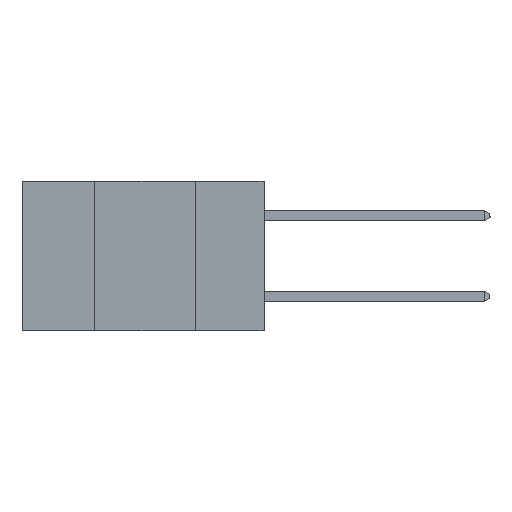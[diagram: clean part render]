
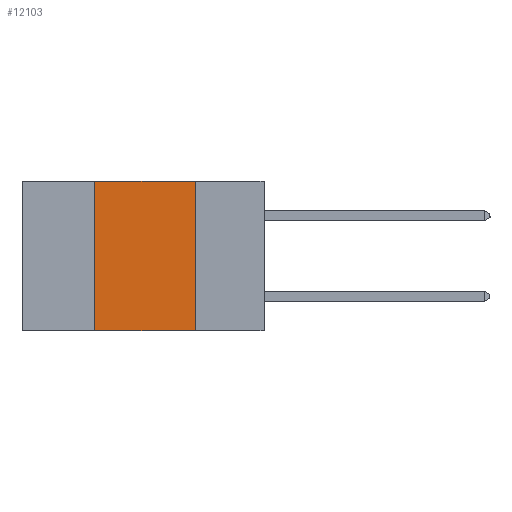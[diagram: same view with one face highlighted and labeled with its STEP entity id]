
A CAD part, left-side view. The second image highlights one B-rep face of the part: STEP entity #12103.
In plain terms, the highlighted planar face has unit normal (-1, 0, 0).
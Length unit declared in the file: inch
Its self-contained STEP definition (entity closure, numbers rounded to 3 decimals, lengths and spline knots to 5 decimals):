
#478 = EDGE_CURVE ( 'NONE', #19204, #480, #9037, .T. ) ;
#480 = VERTEX_POINT ( 'NONE', #11273 ) ;
#606 = CARTESIAN_POINT ( 'NONE',  ( 0., 0.17, -0.37 ) ) ;
#724 = EDGE_CURVE ( 'NONE', #11388, #19204, #14374, .T. ) ;
#988 = FACE_OUTER_BOUND ( 'NONE', #17127, .T. ) ;
#1569 = DIRECTION ( 'NONE',  ( 0., 0., -1. ) ) ;
#3702 = DIRECTION ( 'NONE',  ( 0., -1., 0. ) ) ;
#4059 = VERTEX_POINT ( 'NONE', #606 ) ;
#4669 = VECTOR ( 'NONE', #14485, 39.37008 ) ;
#5579 = EDGE_CURVE ( 'NONE', #480, #4059, #12079, .T. ) ;
#6885 = ORIENTED_EDGE ( 'NONE', *, *, #8822, .T. ) ;
#7453 = VECTOR ( 'NONE', #1569, 39.37008 ) ;
#8600 = PLANE ( 'NONE',  #18018 ) ;
#8822 = EDGE_CURVE ( 'NONE', #11388, #4059, #10202, .T. ) ;
#9037 = LINE ( 'NONE', #18674, #18126 ) ;
#9339 = ORIENTED_EDGE ( 'NONE', *, *, #5579, .F. ) ;
#10202 = LINE ( 'NONE', #10379, #18717 ) ;
#10290 = CARTESIAN_POINT ( 'NONE',  ( 0., 0.17, 0. ) ) ;
#10379 = CARTESIAN_POINT ( 'NONE',  ( 0., 0.6, -0.37 ) ) ;
#11273 = CARTESIAN_POINT ( 'NONE',  ( 0., 0.17, 0. ) ) ;
#11388 = VERTEX_POINT ( 'NONE', #11892 ) ;
#11892 = CARTESIAN_POINT ( 'NONE',  ( 0., 0.42, -0.37 ) ) ;
#12079 = LINE ( 'NONE', #10290, #7453 ) ;
#12091 = DIRECTION ( 'NONE',  ( 0., 0., -1. ) ) ;
#12103 = ADVANCED_FACE ( 'NONE', ( #988 ), #8600, .F. ) ;
#14374 = LINE ( 'NONE', #15922, #4669 ) ;
#14413 = ORIENTED_EDGE ( 'NONE', *, *, #478, .F. ) ;
#14485 = DIRECTION ( 'NONE',  ( 0., 0., 1. ) ) ;
#15499 = ORIENTED_EDGE ( 'NONE', *, *, #724, .F. ) ;
#15922 = CARTESIAN_POINT ( 'NONE',  ( 0., 0.42, 0. ) ) ;
#17127 = EDGE_LOOP ( 'NONE', ( #9339, #14413, #15499, #6885 ) ) ;
#17168 = DIRECTION ( 'NONE',  ( 0., -1., 0. ) ) ;
#18018 = AXIS2_PLACEMENT_3D ( 'NONE', #20556, #22231, #12091 ) ;
#18126 = VECTOR ( 'NONE', #3702, 39.37008 ) ;
#18674 = CARTESIAN_POINT ( 'NONE',  ( 0., 0.6, 0. ) ) ;
#18717 = VECTOR ( 'NONE', #17168, 39.37008 ) ;
#19204 = VERTEX_POINT ( 'NONE', #19633 ) ;
#19633 = CARTESIAN_POINT ( 'NONE',  ( 0., 0.42, 0. ) ) ;
#20556 = CARTESIAN_POINT ( 'NONE',  ( 0., 0.6, 0. ) ) ;
#22231 = DIRECTION ( 'NONE',  ( 1., 0., 0. ) ) ;
